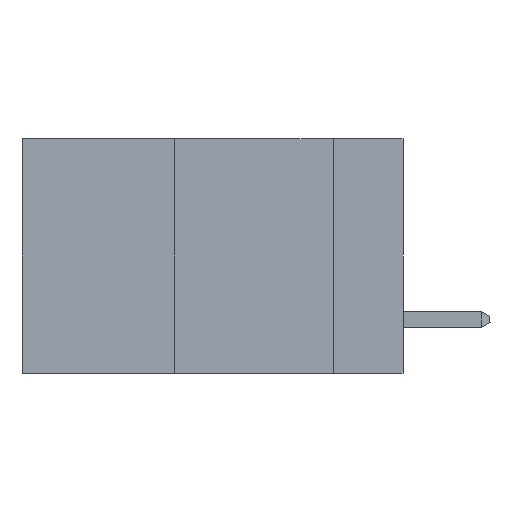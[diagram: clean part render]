
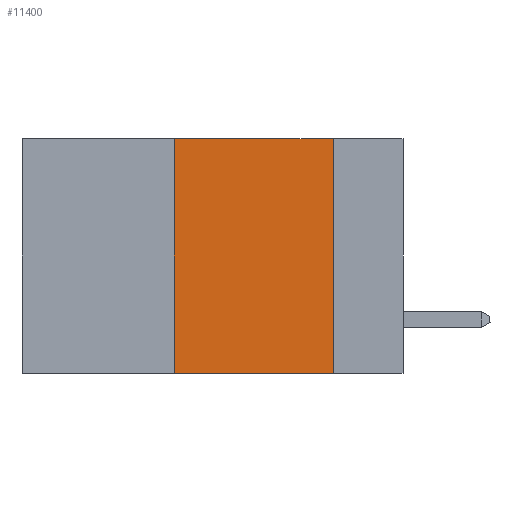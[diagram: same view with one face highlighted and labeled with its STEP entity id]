
A CAD part, left-side view. The second image highlights one B-rep face of the part: STEP entity #11400.
In plain terms, the highlighted planar face has unit normal (-1, 0, 0).
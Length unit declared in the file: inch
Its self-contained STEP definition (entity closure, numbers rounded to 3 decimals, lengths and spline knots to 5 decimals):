
#771 = EDGE_LOOP ( 'NONE', ( #1643, #9695, #14519, #4492 ) ) ;
#1643 = ORIENTED_EDGE ( 'NONE', *, *, #5904, .F. ) ;
#1820 = VECTOR ( 'NONE', #2801, 39.37008 ) ;
#2561 = CARTESIAN_POINT ( 'NONE',  ( 0., 0.11, 0. ) ) ;
#2801 = DIRECTION ( 'NONE',  ( 0., -1., 0. ) ) ;
#2914 = LINE ( 'NONE', #2561, #14856 ) ;
#4137 = CARTESIAN_POINT ( 'NONE',  ( 0., 0.36, 0. ) ) ;
#4338 = EDGE_CURVE ( 'NONE', #4402, #7174, #6802, .T. ) ;
#4402 = VERTEX_POINT ( 'NONE', #5035 ) ;
#4492 = ORIENTED_EDGE ( 'NONE', *, *, #4338, .T. ) ;
#4960 = CARTESIAN_POINT ( 'NONE',  ( 0., 0.6, -0.37 ) ) ;
#5035 = CARTESIAN_POINT ( 'NONE',  ( 0., 0.36, -0.37 ) ) ;
#5074 = PLANE ( 'NONE',  #12884 ) ;
#5661 = VERTEX_POINT ( 'NONE', #8068 ) ;
#5904 = EDGE_CURVE ( 'NONE', #5661, #7174, #2914, .T. ) ;
#5944 = EDGE_CURVE ( 'NONE', #4402, #17673, #17880, .T. ) ;
#6578 = DIRECTION ( 'NONE',  ( 0., 0., -1. ) ) ;
#6802 = LINE ( 'NONE', #4960, #7261 ) ;
#7174 = VERTEX_POINT ( 'NONE', #19243 ) ;
#7261 = VECTOR ( 'NONE', #16886, 39.37008 ) ;
#8068 = CARTESIAN_POINT ( 'NONE',  ( 0., 0.11, 0. ) ) ;
#8605 = DIRECTION ( 'NONE',  ( 0., 0., -1. ) ) ;
#9555 = CARTESIAN_POINT ( 'NONE',  ( 0., 0.6, 0. ) ) ;
#9695 = ORIENTED_EDGE ( 'NONE', *, *, #19323, .F. ) ;
#10022 = CARTESIAN_POINT ( 'NONE',  ( 0., 0.36, 0. ) ) ;
#11400 = ADVANCED_FACE ( 'NONE', ( #14851 ), #5074, .F. ) ;
#11843 = CARTESIAN_POINT ( 'NONE',  ( 0., 0.6, 0. ) ) ;
#12884 = AXIS2_PLACEMENT_3D ( 'NONE', #9555, #15480, #6578 ) ;
#13110 = DIRECTION ( 'NONE',  ( 0., 0., 1. ) ) ;
#13764 = LINE ( 'NONE', #11843, #1820 ) ;
#13932 = VECTOR ( 'NONE', #13110, 39.37008 ) ;
#14519 = ORIENTED_EDGE ( 'NONE', *, *, #5944, .F. ) ;
#14851 = FACE_OUTER_BOUND ( 'NONE', #771, .T. ) ;
#14856 = VECTOR ( 'NONE', #8605, 39.37008 ) ;
#15480 = DIRECTION ( 'NONE',  ( 1., 0., 0. ) ) ;
#16886 = DIRECTION ( 'NONE',  ( 0., -1., 0. ) ) ;
#17673 = VERTEX_POINT ( 'NONE', #10022 ) ;
#17880 = LINE ( 'NONE', #4137, #13932 ) ;
#19243 = CARTESIAN_POINT ( 'NONE',  ( 0., 0.11, -0.37 ) ) ;
#19323 = EDGE_CURVE ( 'NONE', #17673, #5661, #13764, .T. ) ;
